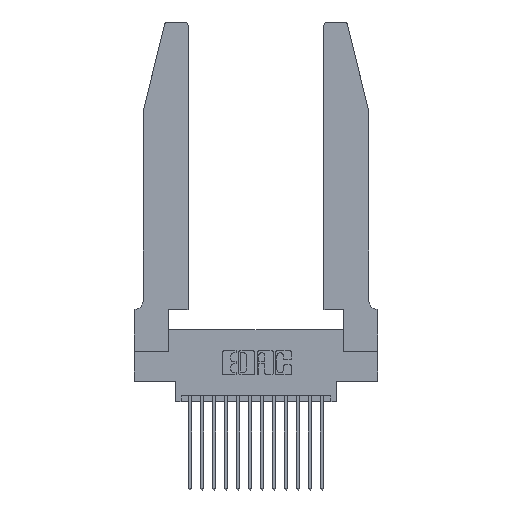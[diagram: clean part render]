
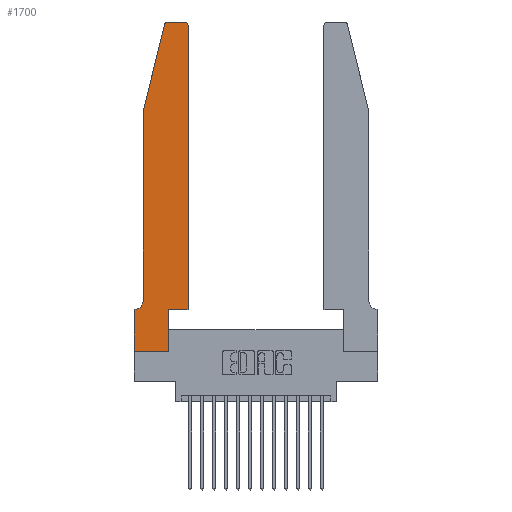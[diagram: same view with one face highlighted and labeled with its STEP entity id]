
A CAD part, top view. The second image highlights one B-rep face of the part: STEP entity #1700.
In plain terms, the highlighted planar face has unit normal (0, 0, 1).
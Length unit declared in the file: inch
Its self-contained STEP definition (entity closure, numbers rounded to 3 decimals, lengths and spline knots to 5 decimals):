
#210 = VECTOR ( 'NONE', #16989, 39.37008 ) ;
#240 = VERTEX_POINT ( 'NONE', #17655 ) ;
#426 = LINE ( 'NONE', #14680, #11809 ) ;
#433 = VERTEX_POINT ( 'NONE', #4670 ) ;
#471 = DIRECTION ( 'NONE',  ( -1., 0., 0. ) ) ;
#530 = EDGE_CURVE ( 'NONE', #8269, #433, #18203, .T. ) ;
#666 = EDGE_CURVE ( 'NONE', #13144, #6088, #8962, .T. ) ;
#673 = CARTESIAN_POINT ( 'NONE',  ( 0.0755, 0.35, 0.37 ) ) ;
#674 = AXIS2_PLACEMENT_3D ( 'NONE', #3012, #12963, #4462 ) ;
#774 = EDGE_CURVE ( 'NONE', #14125, #11919, #7179, .T. ) ;
#825 = CARTESIAN_POINT ( 'NONE',  ( 0.4505, 2.72, 0.37 ) ) ;
#1374 = EDGE_CURVE ( 'NONE', #6088, #240, #11600, .T. ) ;
#1510 = VERTEX_POINT ( 'NONE', #15481 ) ;
#1546 = ORIENTED_EDGE ( 'NONE', *, *, #5658, .T. ) ;
#1585 = EDGE_CURVE ( 'NONE', #2540, #17278, #426, .T. ) ;
#1692 = DIRECTION ( 'NONE',  ( 1., 0., 0. ) ) ;
#1700 = ADVANCED_FACE ( 'NONE', ( #2430 ), #13830, .T. ) ;
#1724 = CARTESIAN_POINT ( 'NONE',  ( 0.4205, 2.72, 0.37 ) ) ;
#1749 = DIRECTION ( 'NONE',  ( 0., 0., 1. ) ) ;
#2349 = DIRECTION ( 'NONE',  ( 0., -1., 0. ) ) ;
#2401 = CARTESIAN_POINT ( 'NONE',  ( 0., 0., 0.37 ) ) ;
#2430 = FACE_OUTER_BOUND ( 'NONE', #17115, .T. ) ;
#2540 = VERTEX_POINT ( 'NONE', #13555 ) ;
#3012 = CARTESIAN_POINT ( 'NONE',  ( 0.0055, 0.42, 0.37 ) ) ;
#3407 = CARTESIAN_POINT ( 'NONE',  ( 0.0755, 2., 0.37 ) ) ;
#3504 = VECTOR ( 'NONE', #2349, 39.37008 ) ;
#3524 = DIRECTION ( 'NONE',  ( 0., 1., 0. ) ) ;
#3569 = DIRECTION ( 'NONE',  ( -0.239, -0.971, 0. ) ) ;
#3714 = CARTESIAN_POINT ( 'NONE',  ( 0.0755, 2., 0.37 ) ) ;
#3746 = CARTESIAN_POINT ( 'NONE',  ( 0.0055, 0.35, 0.37 ) ) ;
#3749 = EDGE_CURVE ( 'NONE', #16133, #13144, #11757, .T. ) ;
#4120 = ORIENTED_EDGE ( 'NONE', *, *, #774, .T. ) ;
#4462 = DIRECTION ( 'NONE',  ( -1., 0., 0. ) ) ;
#4523 = EDGE_CURVE ( 'NONE', #11919, #9242, #14831, .T. ) ;
#4670 = CARTESIAN_POINT ( 'NONE',  ( 0.0755, 2., 0.37 ) ) ;
#4727 = CARTESIAN_POINT ( 'NONE',  ( 0.2865, 0.35, 0.37 ) ) ;
#5076 = EDGE_CURVE ( 'NONE', #433, #1510, #14742, .T. ) ;
#5110 = AXIS2_PLACEMENT_3D ( 'NONE', #15248, #6770, #16642 ) ;
#5521 = ORIENTED_EDGE ( 'NONE', *, *, #3749, .T. ) ;
#5658 = EDGE_CURVE ( 'NONE', #17278, #16133, #6297, .T. ) ;
#5853 = CARTESIAN_POINT ( 'NONE',  ( 0.25487, 2.72718, 0.37 ) ) ;
#5857 = VECTOR ( 'NONE', #13529, 39.37008 ) ;
#6037 = CARTESIAN_POINT ( 'NONE',  ( 0.4205, 2.75, 0.37 ) ) ;
#6088 = VERTEX_POINT ( 'NONE', #6037 ) ;
#6297 = LINE ( 'NONE', #12158, #5857 ) ;
#6467 = LINE ( 'NONE', #2401, #9791 ) ;
#6508 = ORIENTED_EDGE ( 'NONE', *, *, #17637, .T. ) ;
#6591 = DIRECTION ( 'NONE',  ( 0., -1., 0. ) ) ;
#6770 = DIRECTION ( 'NONE',  ( 0., 0., 1. ) ) ;
#6891 = EDGE_CURVE ( 'NONE', #9242, #2540, #6467, .T. ) ;
#7179 = LINE ( 'NONE', #673, #17121 ) ;
#7193 = VECTOR ( 'NONE', #6591, 39.37008 ) ;
#7754 = CARTESIAN_POINT ( 'NONE',  ( 0.4505, 0.35, 0.37 ) ) ;
#8087 = CARTESIAN_POINT ( 'NONE',  ( 0., 0., 0.37 ) ) ;
#8269 = VERTEX_POINT ( 'NONE', #5853 ) ;
#8396 = CARTESIAN_POINT ( 'NONE',  ( 0.4505, 0.35, 0.37 ) ) ;
#8962 = CIRCLE ( 'NONE', #11193, 0.03 ) ;
#9242 = VERTEX_POINT ( 'NONE', #18014 ) ;
#9791 = VECTOR ( 'NONE', #12372, 39.37008 ) ;
#9932 = EDGE_CURVE ( 'NONE', #240, #8269, #15421, .T. ) ;
#10418 = ORIENTED_EDGE ( 'NONE', *, *, #4523, .T. ) ;
#10560 = CARTESIAN_POINT ( 'NONE',  ( 0., 0.35, 0.37 ) ) ;
#11040 = ORIENTED_EDGE ( 'NONE', *, *, #1585, .T. ) ;
#11091 = AXIS2_PLACEMENT_3D ( 'NONE', #13707, #13252, #13229 ) ;
#11193 = AXIS2_PLACEMENT_3D ( 'NONE', #1724, #1749, #1692 ) ;
#11303 = VECTOR ( 'NONE', #3524, 39.37008 ) ;
#11491 = ORIENTED_EDGE ( 'NONE', *, *, #530, .T. ) ;
#11600 = LINE ( 'NONE', #17321, #210 ) ;
#11757 = LINE ( 'NONE', #7754, #11303 ) ;
#11809 = VECTOR ( 'NONE', #14657, 39.37008 ) ;
#11919 = VERTEX_POINT ( 'NONE', #10560 ) ;
#12158 = CARTESIAN_POINT ( 'NONE',  ( 0.4505, 0.35, 0.37 ) ) ;
#12372 = DIRECTION ( 'NONE',  ( 1., 0., 0. ) ) ;
#12963 = DIRECTION ( 'NONE',  ( 0., 0., -1. ) ) ;
#12996 = ORIENTED_EDGE ( 'NONE', *, *, #6891, .T. ) ;
#13144 = VERTEX_POINT ( 'NONE', #825 ) ;
#13172 = ORIENTED_EDGE ( 'NONE', *, *, #5076, .T. ) ;
#13229 = DIRECTION ( 'NONE',  ( 1., 0., 0. ) ) ;
#13252 = DIRECTION ( 'NONE',  ( 0., 0., 1. ) ) ;
#13529 = DIRECTION ( 'NONE',  ( 1., 0., 0. ) ) ;
#13555 = CARTESIAN_POINT ( 'NONE',  ( 0.2865, 0., 0.37 ) ) ;
#13707 = CARTESIAN_POINT ( 'NONE',  ( 0., 0.35, 0.37 ) ) ;
#13830 = PLANE ( 'NONE',  #11091 ) ;
#14054 = VECTOR ( 'NONE', #3569, 39.37008 ) ;
#14125 = VERTEX_POINT ( 'NONE', #3746 ) ;
#14450 = ORIENTED_EDGE ( 'NONE', *, *, #9932, .T. ) ;
#14657 = DIRECTION ( 'NONE',  ( 0., 1., 0. ) ) ;
#14680 = CARTESIAN_POINT ( 'NONE',  ( 0.2865, 0.35, 0.37 ) ) ;
#14742 = LINE ( 'NONE', #3714, #7193 ) ;
#14831 = LINE ( 'NONE', #8087, #3504 ) ;
#15248 = CARTESIAN_POINT ( 'NONE',  ( 0.284, 2.72, 0.37 ) ) ;
#15421 = CIRCLE ( 'NONE', #5110, 0.03 ) ;
#15481 = CARTESIAN_POINT ( 'NONE',  ( 0.0755, 0.42, 0.37 ) ) ;
#16133 = VERTEX_POINT ( 'NONE', #8396 ) ;
#16569 = ORIENTED_EDGE ( 'NONE', *, *, #666, .T. ) ;
#16642 = DIRECTION ( 'NONE',  ( 1., 0., 0. ) ) ;
#16989 = DIRECTION ( 'NONE',  ( -1., 0., 0. ) ) ;
#17115 = EDGE_LOOP ( 'NONE', ( #17511, #14450, #11491, #13172, #6508, #4120, #10418, #12996, #11040, #1546, #5521, #16569 ) ) ;
#17121 = VECTOR ( 'NONE', #471, 39.37008 ) ;
#17186 = CIRCLE ( 'NONE', #674, 0.07 ) ;
#17278 = VERTEX_POINT ( 'NONE', #4727 ) ;
#17321 = CARTESIAN_POINT ( 'NONE',  ( 0.2605, 2.75, 0.37 ) ) ;
#17511 = ORIENTED_EDGE ( 'NONE', *, *, #1374, .T. ) ;
#17637 = EDGE_CURVE ( 'NONE', #1510, #14125, #17186, .T. ) ;
#17655 = CARTESIAN_POINT ( 'NONE',  ( 0.284, 2.75, 0.37 ) ) ;
#18014 = CARTESIAN_POINT ( 'NONE',  ( 0., 0., 0.37 ) ) ;
#18203 = LINE ( 'NONE', #3407, #14054 ) ;
